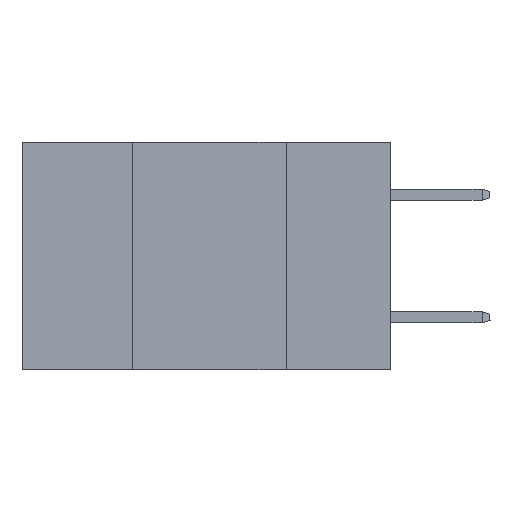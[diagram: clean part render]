
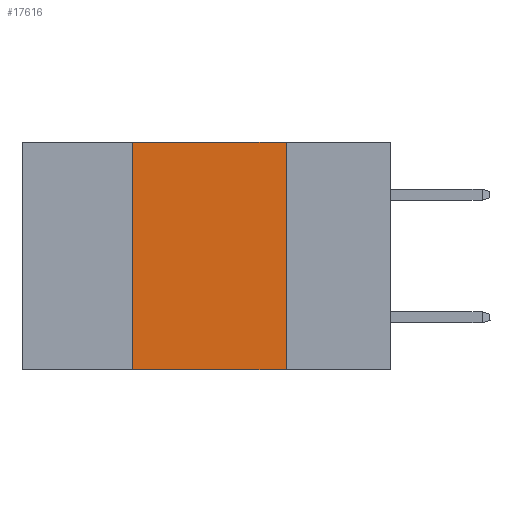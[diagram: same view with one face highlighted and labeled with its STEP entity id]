
A CAD part, left-side view. The second image highlights one B-rep face of the part: STEP entity #17616.
In plain terms, the highlighted planar face has unit normal (-1, 0, 0).
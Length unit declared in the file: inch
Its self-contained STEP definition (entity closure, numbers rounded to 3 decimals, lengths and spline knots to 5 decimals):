
#14 = ORIENTED_EDGE ( 'NONE', *, *, #10184, .T. ) ;
#65 = DIRECTION ( 'NONE',  ( 0., 0., -1. ) ) ;
#631 = CARTESIAN_POINT ( 'NONE',  ( 0., 0.42, 0. ) ) ;
#1013 = DIRECTION ( 'NONE',  ( 0., -1., 0. ) ) ;
#1025 = DIRECTION ( 'NONE',  ( 0., 0., -1. ) ) ;
#1356 = VECTOR ( 'NONE', #1013, 39.37008 ) ;
#1379 = CARTESIAN_POINT ( 'NONE',  ( 0., 0.17, 0. ) ) ;
#2260 = CARTESIAN_POINT ( 'NONE',  ( 0., 0.6, 0. ) ) ;
#2373 = CARTESIAN_POINT ( 'NONE',  ( 0., 0.6, -0.37 ) ) ;
#2610 = FACE_OUTER_BOUND ( 'NONE', #12341, .T. ) ;
#3806 = VERTEX_POINT ( 'NONE', #9368 ) ;
#5028 = CARTESIAN_POINT ( 'NONE',  ( 0., 0.17, -0.37 ) ) ;
#5443 = CARTESIAN_POINT ( 'NONE',  ( 0., 0.42, -0.37 ) ) ;
#5680 = DIRECTION ( 'NONE',  ( 1., 0., 0. ) ) ;
#5945 = ORIENTED_EDGE ( 'NONE', *, *, #8698, .F. ) ;
#6077 = DIRECTION ( 'NONE',  ( 0., 0., 1. ) ) ;
#6805 = CARTESIAN_POINT ( 'NONE',  ( 0., 0.6, 0. ) ) ;
#7105 = EDGE_CURVE ( 'NONE', #7265, #11021, #8120, .T. ) ;
#7265 = VERTEX_POINT ( 'NONE', #1379 ) ;
#8120 = LINE ( 'NONE', #10773, #11043 ) ;
#8175 = PLANE ( 'NONE',  #16518 ) ;
#8411 = VERTEX_POINT ( 'NONE', #5443 ) ;
#8698 = EDGE_CURVE ( 'NONE', #8411, #3806, #14464, .T. ) ;
#8798 = EDGE_CURVE ( 'NONE', #3806, #7265, #15103, .T. ) ;
#9368 = CARTESIAN_POINT ( 'NONE',  ( 0., 0.42, 0. ) ) ;
#10184 = EDGE_CURVE ( 'NONE', #8411, #11021, #16051, .T. ) ;
#10773 = CARTESIAN_POINT ( 'NONE',  ( 0., 0.17, 0. ) ) ;
#10989 = ORIENTED_EDGE ( 'NONE', *, *, #7105, .F. ) ;
#11021 = VERTEX_POINT ( 'NONE', #5028 ) ;
#11043 = VECTOR ( 'NONE', #1025, 39.37008 ) ;
#11123 = VECTOR ( 'NONE', #6077, 39.37008 ) ;
#12008 = DIRECTION ( 'NONE',  ( 0., -1., 0. ) ) ;
#12341 = EDGE_LOOP ( 'NONE', ( #10989, #14226, #5945, #14 ) ) ;
#14226 = ORIENTED_EDGE ( 'NONE', *, *, #8798, .F. ) ;
#14464 = LINE ( 'NONE', #631, #11123 ) ;
#15103 = LINE ( 'NONE', #2260, #17236 ) ;
#16051 = LINE ( 'NONE', #2373, #1356 ) ;
#16518 = AXIS2_PLACEMENT_3D ( 'NONE', #6805, #5680, #65 ) ;
#17236 = VECTOR ( 'NONE', #12008, 39.37008 ) ;
#17616 = ADVANCED_FACE ( 'NONE', ( #2610 ), #8175, .F. ) ;
